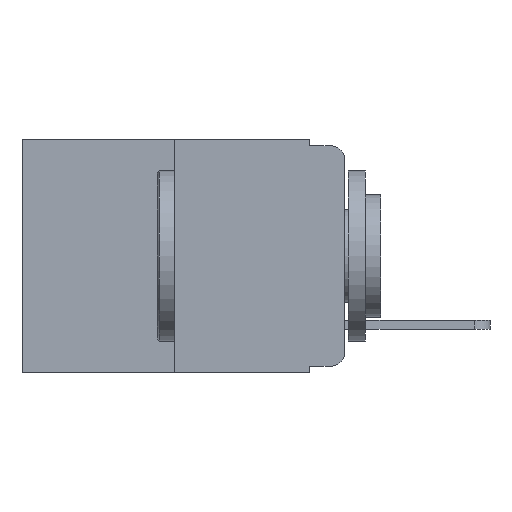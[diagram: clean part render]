
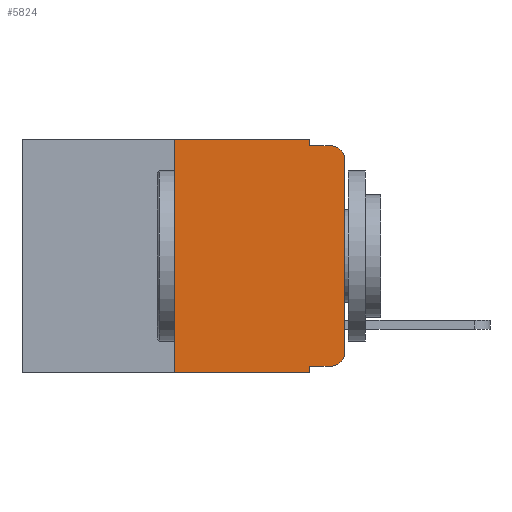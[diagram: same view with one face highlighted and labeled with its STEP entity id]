
A CAD part, left-side view. The second image highlights one B-rep face of the part: STEP entity #5824.
In plain terms, the highlighted planar face has unit normal (-1, 0, 0).
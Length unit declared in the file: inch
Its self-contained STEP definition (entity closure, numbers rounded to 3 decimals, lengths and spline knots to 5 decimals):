
#397 = VECTOR ( 'NONE', #8660, 39.37008 ) ;
#692 = CARTESIAN_POINT ( 'NONE',  ( 0., 0., 0. ) ) ;
#1134 = EDGE_CURVE ( 'NONE', #16485, #1383, #14189, .T. ) ;
#1136 = CARTESIAN_POINT ( 'NONE',  ( 0., 0.25, 0. ) ) ;
#1383 = VERTEX_POINT ( 'NONE', #7934 ) ;
#1521 = PLANE ( 'NONE',  #7242 ) ;
#1819 = VECTOR ( 'NONE', #12391, 39.37008 ) ;
#2132 = EDGE_CURVE ( 'NONE', #21200, #15680, #9124, .T. ) ;
#2247 = VECTOR ( 'NONE', #2913, 39.37008 ) ;
#2913 = DIRECTION ( 'NONE',  ( 0., 0., 1. ) ) ;
#3272 = CARTESIAN_POINT ( 'NONE',  ( 0., 0.02, -0.313 ) ) ;
#3763 = VERTEX_POINT ( 'NONE', #13086 ) ;
#4036 = LINE ( 'NONE', #692, #2247 ) ;
#4060 = CARTESIAN_POINT ( 'NONE',  ( 0., 0.25, -0.343 ) ) ;
#4094 = EDGE_CURVE ( 'NONE', #1383, #3763, #4036, .T. ) ;
#4554 = DIRECTION ( 'NONE',  ( 0., -1., 0. ) ) ;
#4897 = VECTOR ( 'NONE', #4554, 39.37008 ) ;
#5388 = EDGE_CURVE ( 'NONE', #18201, #7631, #18200, .T. ) ;
#5824 = ADVANCED_FACE ( 'NONE', ( #8101 ), #1521, .F. ) ;
#6005 = LINE ( 'NONE', #6666, #1819 ) ;
#6117 = EDGE_CURVE ( 'NONE', #20148, #16485, #16379, .T. ) ;
#6177 = EDGE_LOOP ( 'NONE', ( #19567, #17248, #9032, #13936, #13126, #8268, #19649, #17459, #16403, #20710 ) ) ;
#6198 = EDGE_CURVE ( 'NONE', #10711, #21200, #6005, .T. ) ;
#6666 = CARTESIAN_POINT ( 'NONE',  ( 0., 0.25, 0. ) ) ;
#6959 = DIRECTION ( 'NONE',  ( -1., 0., 0. ) ) ;
#6995 = CARTESIAN_POINT ( 'NONE',  ( 0., 0.473, 0. ) ) ;
#7242 = AXIS2_PLACEMENT_3D ( 'NONE', #24319, #22238, #7443 ) ;
#7443 = DIRECTION ( 'NONE',  ( 0., 0., -1. ) ) ;
#7631 = VERTEX_POINT ( 'NONE', #14624 ) ;
#7834 = CARTESIAN_POINT ( 'NONE',  ( 0., 0.051, -0.01 ) ) ;
#7934 = CARTESIAN_POINT ( 'NONE',  ( 0., 0., -0.313 ) ) ;
#8101 = FACE_OUTER_BOUND ( 'NONE', #6177, .T. ) ;
#8268 = ORIENTED_EDGE ( 'NONE', *, *, #6198, .F. ) ;
#8592 = CARTESIAN_POINT ( 'NONE',  ( 0., 0.473, -0.343 ) ) ;
#8660 = DIRECTION ( 'NONE',  ( 0., 0., -1. ) ) ;
#8727 = DIRECTION ( 'NONE',  ( 0., -1., 0. ) ) ;
#9032 = ORIENTED_EDGE ( 'NONE', *, *, #5388, .F. ) ;
#9124 = LINE ( 'NONE', #6995, #21835 ) ;
#9287 = DIRECTION ( 'NONE',  ( 0., -1., 0. ) ) ;
#9667 = CARTESIAN_POINT ( 'NONE',  ( 0., 0.051, -0.333 ) ) ;
#10693 = AXIS2_PLACEMENT_3D ( 'NONE', #13221, #13131, #16862 ) ;
#10711 = VERTEX_POINT ( 'NONE', #4060 ) ;
#10776 = EDGE_CURVE ( 'NONE', #10711, #22006, #22988, .T. ) ;
#12220 = CARTESIAN_POINT ( 'NONE',  ( 0., 0.051, 0. ) ) ;
#12389 = CARTESIAN_POINT ( 'NONE',  ( 0., 0.051, 0. ) ) ;
#12391 = DIRECTION ( 'NONE',  ( 0., 0., 1. ) ) ;
#12827 = DIRECTION ( 'NONE',  ( 0., 0., -1. ) ) ;
#13086 = CARTESIAN_POINT ( 'NONE',  ( 0., 0., -0.03 ) ) ;
#13126 = ORIENTED_EDGE ( 'NONE', *, *, #2132, .F. ) ;
#13131 = DIRECTION ( 'NONE',  ( -1., 0., 0. ) ) ;
#13221 = CARTESIAN_POINT ( 'NONE',  ( 0., 0.02, -0.03 ) ) ;
#13702 = VECTOR ( 'NONE', #23118, 39.37008 ) ;
#13936 = ORIENTED_EDGE ( 'NONE', *, *, #14969, .F. ) ;
#14189 = CIRCLE ( 'NONE', #21577, 0.02 ) ;
#14252 = CARTESIAN_POINT ( 'NONE',  ( 0., 0.051, 0. ) ) ;
#14624 = CARTESIAN_POINT ( 'NONE',  ( 0., 0.02, -0.01 ) ) ;
#14648 = VECTOR ( 'NONE', #9287, 39.37008 ) ;
#14969 = EDGE_CURVE ( 'NONE', #15680, #18201, #22935, .T. ) ;
#15680 = VERTEX_POINT ( 'NONE', #14252 ) ;
#15753 = CARTESIAN_POINT ( 'NONE',  ( 0., 0.051, -0.333 ) ) ;
#16379 = LINE ( 'NONE', #15753, #13702 ) ;
#16403 = ORIENTED_EDGE ( 'NONE', *, *, #6117, .T. ) ;
#16485 = VERTEX_POINT ( 'NONE', #16708 ) ;
#16650 = EDGE_CURVE ( 'NONE', #20148, #22006, #20119, .T. ) ;
#16708 = CARTESIAN_POINT ( 'NONE',  ( 0., 0.02, -0.333 ) ) ;
#16862 = DIRECTION ( 'NONE',  ( 0., 0., -1. ) ) ;
#17248 = ORIENTED_EDGE ( 'NONE', *, *, #20084, .T. ) ;
#17459 = ORIENTED_EDGE ( 'NONE', *, *, #16650, .F. ) ;
#18044 = VECTOR ( 'NONE', #20005, 39.37008 ) ;
#18200 = LINE ( 'NONE', #20943, #14648 ) ;
#18201 = VERTEX_POINT ( 'NONE', #7834 ) ;
#19567 = ORIENTED_EDGE ( 'NONE', *, *, #4094, .T. ) ;
#19649 = ORIENTED_EDGE ( 'NONE', *, *, #10776, .T. ) ;
#19650 = CIRCLE ( 'NONE', #10693, 0.02 ) ;
#20005 = DIRECTION ( 'NONE',  ( 0., 0., -1. ) ) ;
#20084 = EDGE_CURVE ( 'NONE', #3763, #7631, #19650, .T. ) ;
#20119 = LINE ( 'NONE', #12220, #18044 ) ;
#20148 = VERTEX_POINT ( 'NONE', #9667 ) ;
#20710 = ORIENTED_EDGE ( 'NONE', *, *, #1134, .T. ) ;
#20943 = CARTESIAN_POINT ( 'NONE',  ( 0., 0.051, -0.01 ) ) ;
#21200 = VERTEX_POINT ( 'NONE', #1136 ) ;
#21567 = CARTESIAN_POINT ( 'NONE',  ( 0., 0.051, -0.343 ) ) ;
#21577 = AXIS2_PLACEMENT_3D ( 'NONE', #3272, #6959, #12827 ) ;
#21835 = VECTOR ( 'NONE', #8727, 39.37008 ) ;
#22006 = VERTEX_POINT ( 'NONE', #21567 ) ;
#22238 = DIRECTION ( 'NONE',  ( 1., 0., 0. ) ) ;
#22935 = LINE ( 'NONE', #12389, #397 ) ;
#22988 = LINE ( 'NONE', #8592, #4897 ) ;
#23118 = DIRECTION ( 'NONE',  ( 0., -1., 0. ) ) ;
#24319 = CARTESIAN_POINT ( 'NONE',  ( 0., 0.473, 0. ) ) ;
